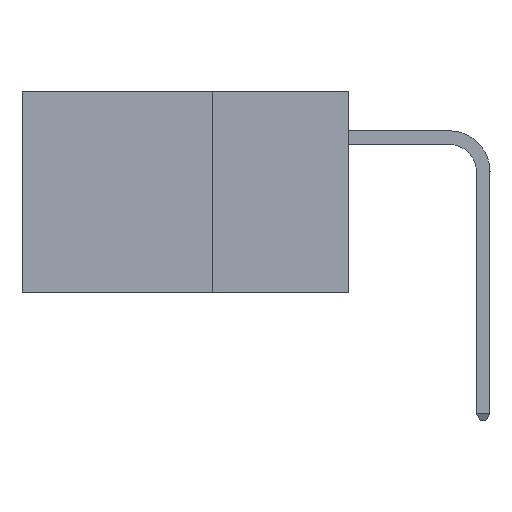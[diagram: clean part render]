
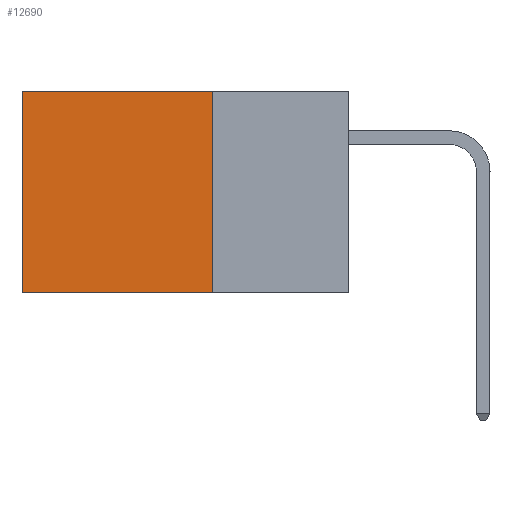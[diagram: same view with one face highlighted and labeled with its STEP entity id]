
A CAD part, left-side view. The second image highlights one B-rep face of the part: STEP entity #12690.
In plain terms, the highlighted planar face has unit normal (-1, 0, 0).
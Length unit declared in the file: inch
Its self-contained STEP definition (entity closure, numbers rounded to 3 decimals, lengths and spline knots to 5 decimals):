
#48 = EDGE_CURVE ( 'NONE', #23850, #18022, #26929, .T. ) ;
#443 = CARTESIAN_POINT ( 'NONE',  ( 0.2875, 0.6, 0. ) ) ;
#3810 = EDGE_LOOP ( 'NONE', ( #7343, #10956, #9546, #20879 ) ) ;
#6499 = DIRECTION ( 'NONE',  ( 0., 0., -1. ) ) ;
#7343 = ORIENTED_EDGE ( 'NONE', *, *, #22312, .T. ) ;
#7498 = DIRECTION ( 'NONE',  ( 0., 1., 0. ) ) ;
#7579 = EDGE_CURVE ( 'NONE', #18022, #13807, #28221, .T. ) ;
#8962 = LINE ( 'NONE', #27076, #19465 ) ;
#9546 = ORIENTED_EDGE ( 'NONE', *, *, #48, .F. ) ;
#9942 = LINE ( 'NONE', #23206, #27092 ) ;
#10956 = ORIENTED_EDGE ( 'NONE', *, *, #7579, .F. ) ;
#11020 = FACE_OUTER_BOUND ( 'NONE', #3810, .T. ) ;
#11031 = PLANE ( 'NONE',  #20774 ) ;
#11223 = CARTESIAN_POINT ( 'NONE',  ( 0.2875, 0.25, -0.37 ) ) ;
#11742 = CARTESIAN_POINT ( 'NONE',  ( 0.2875, 0.25, 0. ) ) ;
#12690 = ADVANCED_FACE ( 'NONE', ( #11020 ), #11031, .F. ) ;
#13591 = EDGE_CURVE ( 'NONE', #23850, #23086, #9942, .T. ) ;
#13738 = DIRECTION ( 'NONE',  ( 0., 0., -1. ) ) ;
#13807 = VERTEX_POINT ( 'NONE', #17761 ) ;
#15583 = DIRECTION ( 'NONE',  ( 0., 0., -1. ) ) ;
#16999 = CARTESIAN_POINT ( 'NONE',  ( 0.2875, 0.25, -0.37 ) ) ;
#17761 = CARTESIAN_POINT ( 'NONE',  ( 0.2875, 0.6, -0.37 ) ) ;
#18022 = VERTEX_POINT ( 'NONE', #16999 ) ;
#19465 = VECTOR ( 'NONE', #13738, 39.37008 ) ;
#20228 = DIRECTION ( 'NONE',  ( 0., 1., 0. ) ) ;
#20774 = AXIS2_PLACEMENT_3D ( 'NONE', #26679, #28917, #15583 ) ;
#20879 = ORIENTED_EDGE ( 'NONE', *, *, #13591, .T. ) ;
#22300 = VECTOR ( 'NONE', #20228, 39.37008 ) ;
#22312 = EDGE_CURVE ( 'NONE', #23086, #13807, #8962, .T. ) ;
#23086 = VERTEX_POINT ( 'NONE', #443 ) ;
#23206 = CARTESIAN_POINT ( 'NONE',  ( 0.2875, 0.25, 0. ) ) ;
#23850 = VERTEX_POINT ( 'NONE', #28327 ) ;
#26219 = VECTOR ( 'NONE', #6499, 39.37008 ) ;
#26679 = CARTESIAN_POINT ( 'NONE',  ( 0.2875, 0.25, 0. ) ) ;
#26929 = LINE ( 'NONE', #11742, #26219 ) ;
#27076 = CARTESIAN_POINT ( 'NONE',  ( 0.2875, 0.6, 0. ) ) ;
#27092 = VECTOR ( 'NONE', #7498, 39.37008 ) ;
#28221 = LINE ( 'NONE', #11223, #22300 ) ;
#28327 = CARTESIAN_POINT ( 'NONE',  ( 0.2875, 0.25, 0. ) ) ;
#28917 = DIRECTION ( 'NONE',  ( 1., 0., 0. ) ) ;
